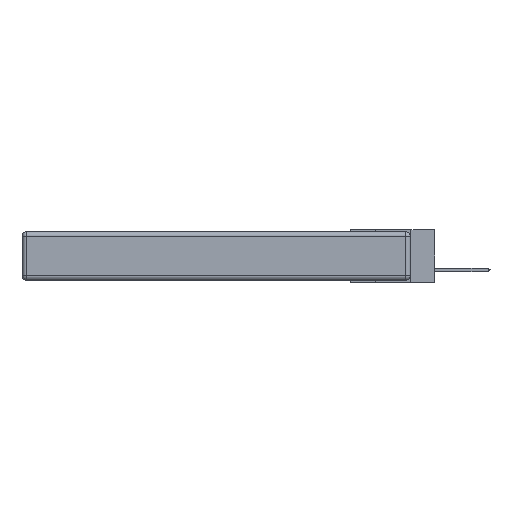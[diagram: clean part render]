
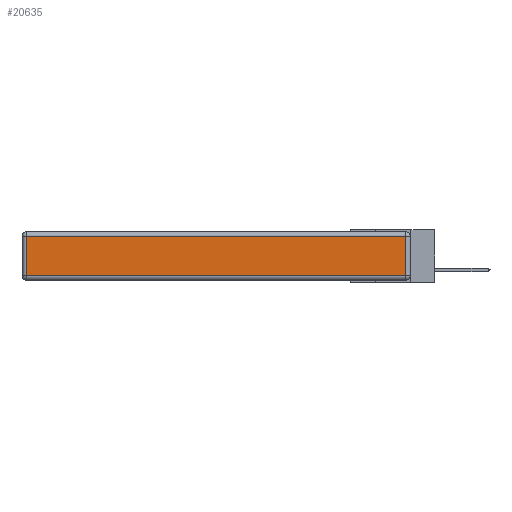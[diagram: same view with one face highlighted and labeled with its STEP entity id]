
A CAD part, left-side view. The second image highlights one B-rep face of the part: STEP entity #20635.
In plain terms, the highlighted planar face has unit normal (-1, 0, 0).
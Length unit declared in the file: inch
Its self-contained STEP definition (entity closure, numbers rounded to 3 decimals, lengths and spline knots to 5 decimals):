
#257 = VECTOR ( 'NONE', #15250, 39.37008 ) ;
#582 = ORIENTED_EDGE ( 'NONE', *, *, #6977, .T. ) ;
#810 = CARTESIAN_POINT ( 'NONE',  ( 0., 0.03, -0.343 ) ) ;
#889 = DIRECTION ( 'NONE',  ( -1., 0., 0. ) ) ;
#1169 = VERTEX_POINT ( 'NONE', #19306 ) ;
#2514 = DIRECTION ( 'NONE',  ( 0., 0., 1. ) ) ;
#3084 = CARTESIAN_POINT ( 'NONE',  ( 0., 2.72, -0.343 ) ) ;
#3103 = ORIENTED_EDGE ( 'NONE', *, *, #13984, .T. ) ;
#4219 = CARTESIAN_POINT ( 'NONE',  ( 0., 0., -0.343 ) ) ;
#4349 = LINE ( 'NONE', #15827, #16836 ) ;
#4430 = CARTESIAN_POINT ( 'NONE',  ( 0., 0.03, -0.03 ) ) ;
#4577 = VERTEX_POINT ( 'NONE', #17343 ) ;
#5206 = EDGE_CURVE ( 'NONE', #13513, #5220, #8779, .T. ) ;
#5220 = VERTEX_POINT ( 'NONE', #4430 ) ;
#5674 = PLANE ( 'NONE',  #13333 ) ;
#6340 = ORIENTED_EDGE ( 'NONE', *, *, #5206, .T. ) ;
#6977 = EDGE_CURVE ( 'NONE', #5220, #1169, #12752, .T. ) ;
#7132 = EDGE_LOOP ( 'NONE', ( #16542, #6340, #582, #3103 ) ) ;
#8779 = LINE ( 'NONE', #810, #13310 ) ;
#9337 = DIRECTION ( 'NONE',  ( 0., 0., -1. ) ) ;
#10127 = LINE ( 'NONE', #3084, #20588 ) ;
#11014 = EDGE_CURVE ( 'NONE', #4577, #13513, #4349, .T. ) ;
#12000 = DIRECTION ( 'NONE',  ( 0., 0., 1. ) ) ;
#12752 = LINE ( 'NONE', #18352, #257 ) ;
#13310 = VECTOR ( 'NONE', #2514, 39.37008 ) ;
#13333 = AXIS2_PLACEMENT_3D ( 'NONE', #4219, #889, #12000 ) ;
#13513 = VERTEX_POINT ( 'NONE', #15341 ) ;
#13984 = EDGE_CURVE ( 'NONE', #1169, #4577, #10127, .T. ) ;
#14407 = DIRECTION ( 'NONE',  ( 0., -1., 0. ) ) ;
#15250 = DIRECTION ( 'NONE',  ( 0., 1., 0. ) ) ;
#15341 = CARTESIAN_POINT ( 'NONE',  ( 0., 0.03, -0.313 ) ) ;
#15827 = CARTESIAN_POINT ( 'NONE',  ( 0., 0., -0.313 ) ) ;
#16542 = ORIENTED_EDGE ( 'NONE', *, *, #11014, .T. ) ;
#16836 = VECTOR ( 'NONE', #14407, 39.37008 ) ;
#17343 = CARTESIAN_POINT ( 'NONE',  ( 0., 2.72, -0.313 ) ) ;
#18352 = CARTESIAN_POINT ( 'NONE',  ( 0., 2.75, -0.03 ) ) ;
#19089 = FACE_OUTER_BOUND ( 'NONE', #7132, .T. ) ;
#19306 = CARTESIAN_POINT ( 'NONE',  ( 0., 2.72, -0.03 ) ) ;
#20588 = VECTOR ( 'NONE', #9337, 39.37008 ) ;
#20635 = ADVANCED_FACE ( 'NONE', ( #19089 ), #5674, .T. ) ;
